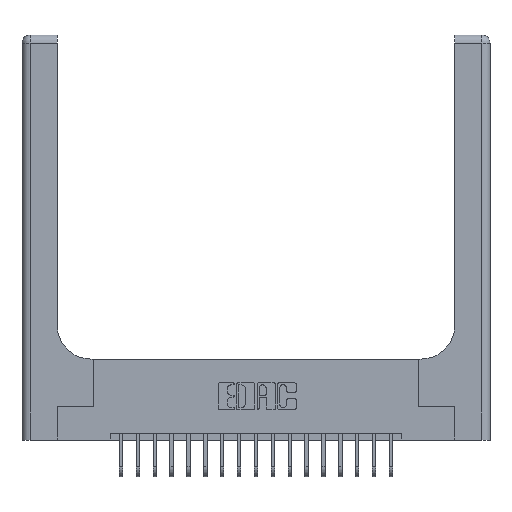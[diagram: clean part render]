
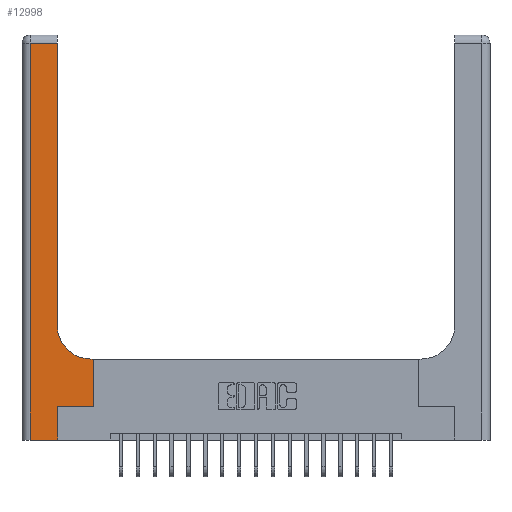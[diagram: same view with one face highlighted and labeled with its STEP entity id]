
A CAD part, top view. The second image highlights one B-rep face of the part: STEP entity #12998.
In plain terms, the highlighted planar face has unit normal (0, 0, 1).
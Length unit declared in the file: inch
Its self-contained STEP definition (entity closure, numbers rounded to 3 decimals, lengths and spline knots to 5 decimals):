
#40 = DIRECTION ( 'NONE',  ( -1., 0., 0. ) ) ;
#222 = ORIENTED_EDGE ( 'NONE', *, *, #11818, .T. ) ;
#262 = DIRECTION ( 'NONE',  ( -1., 0., 0. ) ) ;
#863 = LINE ( 'NONE', #6942, #11770 ) ;
#1091 = ORIENTED_EDGE ( 'NONE', *, *, #11259, .T. ) ;
#2370 = VERTEX_POINT ( 'NONE', #8045 ) ;
#2479 = CARTESIAN_POINT ( 'NONE',  ( 0., 2.94, 0.37 ) ) ;
#2552 = DIRECTION ( 'NONE',  ( -1., 0., 0. ) ) ;
#2566 = VECTOR ( 'NONE', #12272, 39.37008 ) ;
#2585 = VERTEX_POINT ( 'NONE', #3813 ) ;
#3493 = DIRECTION ( 'NONE',  ( 0., 1., 0. ) ) ;
#3624 = VECTOR ( 'NONE', #21191, 39.37008 ) ;
#3813 = CARTESIAN_POINT ( 'NONE',  ( 0.51, 0.6, 0.37 ) ) ;
#4059 = VERTEX_POINT ( 'NONE', #12003 ) ;
#4154 = ORIENTED_EDGE ( 'NONE', *, *, #18423, .T. ) ;
#4604 = VERTEX_POINT ( 'NONE', #15004 ) ;
#4802 = EDGE_CURVE ( 'NONE', #2585, #7070, #5822, .T. ) ;
#4944 = CARTESIAN_POINT ( 'NONE',  ( 0.528, 0.25, 0.37 ) ) ;
#5006 = PLANE ( 'NONE',  #15176 ) ;
#5214 = CARTESIAN_POINT ( 'NONE',  ( 0., 3., 0.37 ) ) ;
#5822 = CIRCLE ( 'NONE', #10661, 0.25 ) ;
#5828 = EDGE_CURVE ( 'NONE', #10581, #14207, #6326, .T. ) ;
#6167 = LINE ( 'NONE', #17038, #2566 ) ;
#6326 = LINE ( 'NONE', #4944, #9713 ) ;
#6586 = ORIENTED_EDGE ( 'NONE', *, *, #13234, .T. ) ;
#6942 = CARTESIAN_POINT ( 'NONE',  ( 0.265, 0.25, 0.37 ) ) ;
#7070 = VERTEX_POINT ( 'NONE', #11245 ) ;
#7450 = DIRECTION ( 'NONE',  ( 0., 0., -1. ) ) ;
#7596 = DIRECTION ( 'NONE',  ( 1., 0., 0. ) ) ;
#8033 = LINE ( 'NONE', #8097, #18428 ) ;
#8045 = CARTESIAN_POINT ( 'NONE',  ( 0.26, 2.94, 0.37 ) ) ;
#8097 = CARTESIAN_POINT ( 'NONE',  ( 0.26, 0.6, 0.37 ) ) ;
#8297 = DIRECTION ( 'NONE',  ( 0., 0., -1. ) ) ;
#9184 = VECTOR ( 'NONE', #16476, 39.37008 ) ;
#9206 = ORIENTED_EDGE ( 'NONE', *, *, #5828, .T. ) ;
#9650 = CARTESIAN_POINT ( 'NONE',  ( 0.265, 0.25, 0.37 ) ) ;
#9713 = VECTOR ( 'NONE', #3493, 39.37008 ) ;
#10231 = VERTEX_POINT ( 'NONE', #9650 ) ;
#10581 = VERTEX_POINT ( 'NONE', #12029 ) ;
#10661 = AXIS2_PLACEMENT_3D ( 'NONE', #17676, #7450, #7596 ) ;
#10916 = CARTESIAN_POINT ( 'NONE',  ( 0.265, 0., 0.37 ) ) ;
#10986 = EDGE_CURVE ( 'NONE', #14207, #2585, #8033, .T. ) ;
#11245 = CARTESIAN_POINT ( 'NONE',  ( 0.26, 0.85, 0.37 ) ) ;
#11259 = EDGE_CURVE ( 'NONE', #4604, #10231, #19434, .T. ) ;
#11508 = CARTESIAN_POINT ( 'NONE',  ( 0., 0., 0.37 ) ) ;
#11770 = VECTOR ( 'NONE', #18499, 39.37008 ) ;
#11818 = EDGE_CURVE ( 'NONE', #7070, #2370, #6167, .T. ) ;
#12003 = CARTESIAN_POINT ( 'NONE',  ( 0.06, 0., 0.37 ) ) ;
#12029 = CARTESIAN_POINT ( 'NONE',  ( 0.528, 0.25, 0.37 ) ) ;
#12272 = DIRECTION ( 'NONE',  ( 0., 1., 0. ) ) ;
#12434 = DIRECTION ( 'NONE',  ( 0., 1., 0. ) ) ;
#12998 = ADVANCED_FACE ( 'NONE', ( #14937 ), #5006, .F. ) ;
#13101 = CARTESIAN_POINT ( 'NONE',  ( 0.528, 0.6, 0.37 ) ) ;
#13234 = EDGE_CURVE ( 'NONE', #2370, #16869, #19875, .T. ) ;
#13579 = LINE ( 'NONE', #11508, #9184 ) ;
#14207 = VERTEX_POINT ( 'NONE', #13101 ) ;
#14522 = CARTESIAN_POINT ( 'NONE',  ( 0.06, 3., 0.37 ) ) ;
#14600 = ORIENTED_EDGE ( 'NONE', *, *, #16946, .T. ) ;
#14651 = EDGE_CURVE ( 'NONE', #4059, #4604, #13579, .T. ) ;
#14937 = FACE_OUTER_BOUND ( 'NONE', #20058, .T. ) ;
#15004 = CARTESIAN_POINT ( 'NONE',  ( 0.265, 0., 0.37 ) ) ;
#15176 = AXIS2_PLACEMENT_3D ( 'NONE', #5214, #8297, #40 ) ;
#15421 = ORIENTED_EDGE ( 'NONE', *, *, #10986, .T. ) ;
#16376 = CARTESIAN_POINT ( 'NONE',  ( 0.06, 2.94, 0.37 ) ) ;
#16476 = DIRECTION ( 'NONE',  ( 1., 0., 0. ) ) ;
#16869 = VERTEX_POINT ( 'NONE', #16376 ) ;
#16946 = EDGE_CURVE ( 'NONE', #10231, #10581, #863, .T. ) ;
#17038 = CARTESIAN_POINT ( 'NONE',  ( 0.26, 3., 0.37 ) ) ;
#17060 = ORIENTED_EDGE ( 'NONE', *, *, #14651, .T. ) ;
#17676 = CARTESIAN_POINT ( 'NONE',  ( 0.51, 0.85, 0.37 ) ) ;
#18423 = EDGE_CURVE ( 'NONE', #16869, #4059, #18954, .T. ) ;
#18428 = VECTOR ( 'NONE', #262, 39.37008 ) ;
#18499 = DIRECTION ( 'NONE',  ( 1., 0., 0. ) ) ;
#18954 = LINE ( 'NONE', #14522, #3624 ) ;
#19434 = LINE ( 'NONE', #10916, #21228 ) ;
#19875 = LINE ( 'NONE', #2479, #21417 ) ;
#20058 = EDGE_LOOP ( 'NONE', ( #222, #6586, #4154, #17060, #1091, #14600, #9206, #15421, #21040 ) ) ;
#21040 = ORIENTED_EDGE ( 'NONE', *, *, #4802, .T. ) ;
#21191 = DIRECTION ( 'NONE',  ( 0., -1., 0. ) ) ;
#21228 = VECTOR ( 'NONE', #12434, 39.37008 ) ;
#21417 = VECTOR ( 'NONE', #2552, 39.37008 ) ;
